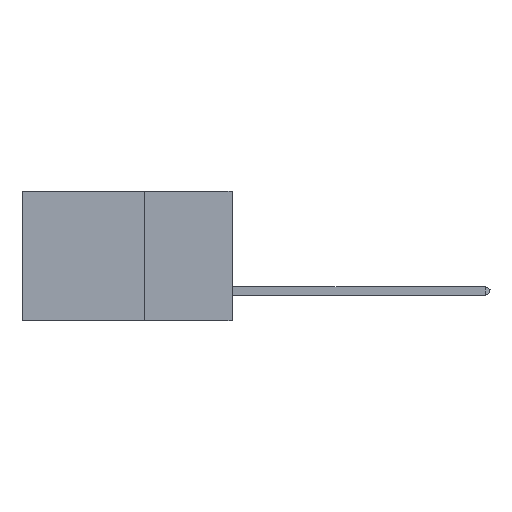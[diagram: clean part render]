
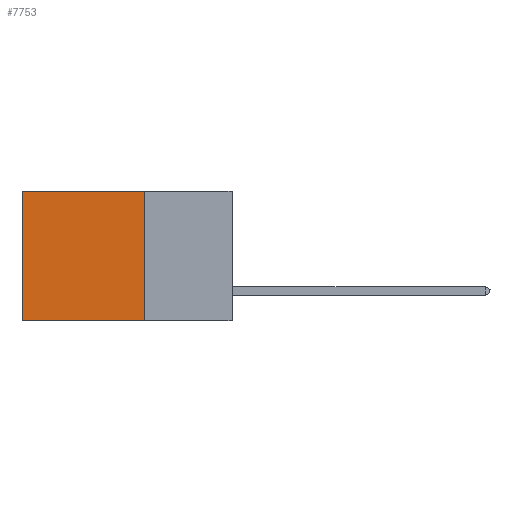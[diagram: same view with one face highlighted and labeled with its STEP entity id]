
A CAD part, left-side view. The second image highlights one B-rep face of the part: STEP entity #7753.
In plain terms, the highlighted planar face has unit normal (-1, 0, 0).
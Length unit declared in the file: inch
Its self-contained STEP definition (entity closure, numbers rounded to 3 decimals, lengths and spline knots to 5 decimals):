
#559 = VECTOR ( 'NONE', #10902, 39.37008 ) ;
#662 = VERTEX_POINT ( 'NONE', #1636 ) ;
#997 = CARTESIAN_POINT ( 'NONE',  ( 0.2875, 0.25, 0. ) ) ;
#1636 = CARTESIAN_POINT ( 'NONE',  ( 0.2875, 0.25, 0. ) ) ;
#2620 = CARTESIAN_POINT ( 'NONE',  ( 0.2875, 0.25, -0.37 ) ) ;
#2722 = DIRECTION ( 'NONE',  ( 0., 0., -1. ) ) ;
#2781 = DIRECTION ( 'NONE',  ( 0., 1., 0. ) ) ;
#3783 = VECTOR ( 'NONE', #20831, 39.37008 ) ;
#4065 = CARTESIAN_POINT ( 'NONE',  ( 0.2875, 0.25, 0. ) ) ;
#4180 = VERTEX_POINT ( 'NONE', #14760 ) ;
#4331 = LINE ( 'NONE', #8525, #3783 ) ;
#4533 = DIRECTION ( 'NONE',  ( 1., 0., 0. ) ) ;
#4819 = VECTOR ( 'NONE', #2781, 39.37008 ) ;
#5433 = EDGE_CURVE ( 'NONE', #13774, #21720, #4331, .T. ) ;
#7753 = ADVANCED_FACE ( 'NONE', ( #11908 ), #8159, .F. ) ;
#7758 = LINE ( 'NONE', #21296, #15167 ) ;
#7846 = ORIENTED_EDGE ( 'NONE', *, *, #21651, .F. ) ;
#7970 = CARTESIAN_POINT ( 'NONE',  ( 0.2875, 0.6, -0.37 ) ) ;
#8159 = PLANE ( 'NONE',  #8758 ) ;
#8521 = EDGE_LOOP ( 'NONE', ( #8995, #7846, #9353, #17912 ) ) ;
#8525 = CARTESIAN_POINT ( 'NONE',  ( 0.2875, 0.6, 0. ) ) ;
#8758 = AXIS2_PLACEMENT_3D ( 'NONE', #997, #4533, #2722 ) ;
#8946 = EDGE_CURVE ( 'NONE', #662, #13774, #7758, .T. ) ;
#8995 = ORIENTED_EDGE ( 'NONE', *, *, #5433, .T. ) ;
#9353 = ORIENTED_EDGE ( 'NONE', *, *, #16556, .F. ) ;
#10902 = DIRECTION ( 'NONE',  ( 0., 0., -1. ) ) ;
#11908 = FACE_OUTER_BOUND ( 'NONE', #8521, .T. ) ;
#11973 = LINE ( 'NONE', #2620, #4819 ) ;
#13774 = VERTEX_POINT ( 'NONE', #22276 ) ;
#14760 = CARTESIAN_POINT ( 'NONE',  ( 0.2875, 0.25, -0.37 ) ) ;
#15167 = VECTOR ( 'NONE', #16018, 39.37008 ) ;
#16018 = DIRECTION ( 'NONE',  ( 0., 1., 0. ) ) ;
#16556 = EDGE_CURVE ( 'NONE', #662, #4180, #18740, .T. ) ;
#17912 = ORIENTED_EDGE ( 'NONE', *, *, #8946, .T. ) ;
#18740 = LINE ( 'NONE', #4065, #559 ) ;
#20831 = DIRECTION ( 'NONE',  ( 0., 0., -1. ) ) ;
#21296 = CARTESIAN_POINT ( 'NONE',  ( 0.2875, 0.25, 0. ) ) ;
#21651 = EDGE_CURVE ( 'NONE', #4180, #21720, #11973, .T. ) ;
#21720 = VERTEX_POINT ( 'NONE', #7970 ) ;
#22276 = CARTESIAN_POINT ( 'NONE',  ( 0.2875, 0.6, 0. ) ) ;
